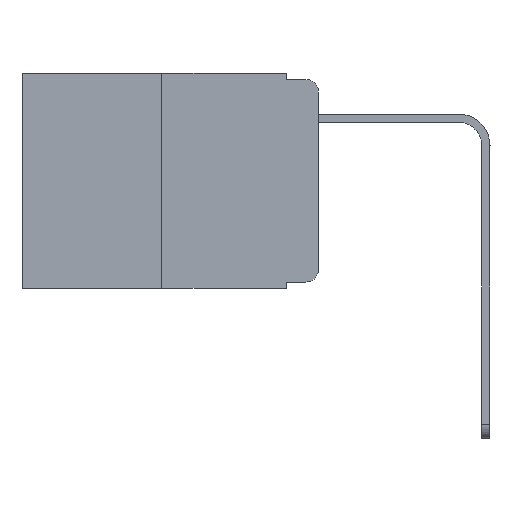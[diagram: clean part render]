
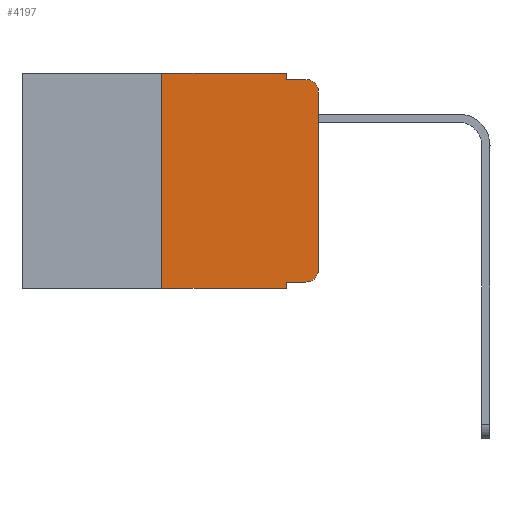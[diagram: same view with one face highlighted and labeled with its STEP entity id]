
A CAD part, left-side view. The second image highlights one B-rep face of the part: STEP entity #4197.
In plain terms, the highlighted planar face has unit normal (-1, 0, 0).
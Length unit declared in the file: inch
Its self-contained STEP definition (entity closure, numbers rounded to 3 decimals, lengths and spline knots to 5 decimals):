
#75 = VERTEX_POINT ( 'NONE', #1834 ) ;
#324 = VERTEX_POINT ( 'NONE', #2211 ) ;
#340 = ORIENTED_EDGE ( 'NONE', *, *, #642, .T. ) ;
#403 = DIRECTION ( 'NONE',  ( -1., 0., 0. ) ) ;
#424 = DIRECTION ( 'NONE',  ( 0., 0., -1. ) ) ;
#642 = EDGE_CURVE ( 'NONE', #324, #2455, #707, .T. ) ;
#693 = CARTESIAN_POINT ( 'NONE',  ( 0., 0.02, -0.01 ) ) ;
#707 = CIRCLE ( 'NONE', #5364, 0.02 ) ;
#715 = DIRECTION ( 'NONE',  ( 0., 0., 1. ) ) ;
#959 = CARTESIAN_POINT ( 'NONE',  ( 0., 0.25, 0. ) ) ;
#1216 = VECTOR ( 'NONE', #8042, 39.37008 ) ;
#1323 = DIRECTION ( 'NONE',  ( 0., -1., 0. ) ) ;
#1361 = CARTESIAN_POINT ( 'NONE',  ( 0., 0.473, -0.343 ) ) ;
#1696 = EDGE_CURVE ( 'NONE', #6298, #324, #5935, .T. ) ;
#1725 = VECTOR ( 'NONE', #3395, 39.37008 ) ;
#1813 = VERTEX_POINT ( 'NONE', #959 ) ;
#1834 = CARTESIAN_POINT ( 'NONE',  ( 0., 0.25, -0.343 ) ) ;
#2011 = CARTESIAN_POINT ( 'NONE',  ( 0., 0.25, 0. ) ) ;
#2147 = VERTEX_POINT ( 'NONE', #693 ) ;
#2211 = CARTESIAN_POINT ( 'NONE',  ( 0., 0.02, -0.333 ) ) ;
#2455 = VERTEX_POINT ( 'NONE', #8117 ) ;
#2466 = EDGE_CURVE ( 'NONE', #11154, #2147, #7695, .T. ) ;
#2518 = VERTEX_POINT ( 'NONE', #2877 ) ;
#2546 = LINE ( 'NONE', #7558, #6874 ) ;
#2628 = LINE ( 'NONE', #1361, #7210 ) ;
#2637 = VECTOR ( 'NONE', #4502, 39.37008 ) ;
#2770 = DIRECTION ( 'NONE',  ( 0., 0., -1. ) ) ;
#2814 = CARTESIAN_POINT ( 'NONE',  ( 0., 0.051, -0.01 ) ) ;
#2847 = EDGE_CURVE ( 'NONE', #2455, #2518, #2546, .T. ) ;
#2877 = CARTESIAN_POINT ( 'NONE',  ( 0., 0., -0.03 ) ) ;
#2889 = ORIENTED_EDGE ( 'NONE', *, *, #3405, .T. ) ;
#2985 = PLANE ( 'NONE',  #8732 ) ;
#3023 = LINE ( 'NONE', #6468, #9498 ) ;
#3395 = DIRECTION ( 'NONE',  ( 0., 0., -1. ) ) ;
#3405 = EDGE_CURVE ( 'NONE', #2518, #2147, #7803, .T. ) ;
#3436 = ORIENTED_EDGE ( 'NONE', *, *, #7038, .F. ) ;
#3482 = LINE ( 'NONE', #8579, #1725 ) ;
#3549 = EDGE_CURVE ( 'NONE', #10260, #11154, #3482, .T. ) ;
#3583 = DIRECTION ( 'NONE',  ( 0., 0., -1. ) ) ;
#3618 = VECTOR ( 'NONE', #6072, 39.37008 ) ;
#3817 = CARTESIAN_POINT ( 'NONE',  ( 0., 0.051, -0.01 ) ) ;
#3830 = CARTESIAN_POINT ( 'NONE',  ( 0., 0.473, 0. ) ) ;
#3977 = CARTESIAN_POINT ( 'NONE',  ( 0., 0.051, -0.343 ) ) ;
#4197 = ADVANCED_FACE ( 'NONE', ( #4848 ), #2985, .F. ) ;
#4306 = CARTESIAN_POINT ( 'NONE',  ( 0., 0.051, -0.333 ) ) ;
#4502 = DIRECTION ( 'NONE',  ( 0., 0., 1. ) ) ;
#4652 = LINE ( 'NONE', #2011, #2637 ) ;
#4848 = FACE_OUTER_BOUND ( 'NONE', #9367, .T. ) ;
#4868 = CARTESIAN_POINT ( 'NONE',  ( 0., 0.051, -0.333 ) ) ;
#4989 = ORIENTED_EDGE ( 'NONE', *, *, #2466, .F. ) ;
#5224 = EDGE_CURVE ( 'NONE', #6298, #9052, #8194, .T. ) ;
#5237 = ORIENTED_EDGE ( 'NONE', *, *, #10431, .F. ) ;
#5251 = DIRECTION ( 'NONE',  ( -1., 0., 0. ) ) ;
#5364 = AXIS2_PLACEMENT_3D ( 'NONE', #9698, #5251, #3583 ) ;
#5935 = LINE ( 'NONE', #4306, #3618 ) ;
#6072 = DIRECTION ( 'NONE',  ( 0., -1., 0. ) ) ;
#6174 = VECTOR ( 'NONE', #2770, 39.37008 ) ;
#6298 = VERTEX_POINT ( 'NONE', #4868 ) ;
#6468 = CARTESIAN_POINT ( 'NONE',  ( 0., 0.473, 0. ) ) ;
#6860 = ORIENTED_EDGE ( 'NONE', *, *, #1696, .T. ) ;
#6874 = VECTOR ( 'NONE', #715, 39.37008 ) ;
#7038 = EDGE_CURVE ( 'NONE', #75, #1813, #4652, .T. ) ;
#7210 = VECTOR ( 'NONE', #9217, 39.37008 ) ;
#7366 = ORIENTED_EDGE ( 'NONE', *, *, #2847, .T. ) ;
#7558 = CARTESIAN_POINT ( 'NONE',  ( 0., 0., 0. ) ) ;
#7695 = LINE ( 'NONE', #2814, #1216 ) ;
#7803 = CIRCLE ( 'NONE', #8286, 0.02 ) ;
#7929 = CARTESIAN_POINT ( 'NONE',  ( 0., 0.051, 0. ) ) ;
#7945 = CARTESIAN_POINT ( 'NONE',  ( 0., 0.051, 0. ) ) ;
#8037 = CARTESIAN_POINT ( 'NONE',  ( 0., 0.02, -0.03 ) ) ;
#8042 = DIRECTION ( 'NONE',  ( 0., -1., 0. ) ) ;
#8117 = CARTESIAN_POINT ( 'NONE',  ( 0., 0., -0.313 ) ) ;
#8194 = LINE ( 'NONE', #7929, #6174 ) ;
#8247 = EDGE_CURVE ( 'NONE', #75, #9052, #2628, .T. ) ;
#8286 = AXIS2_PLACEMENT_3D ( 'NONE', #8037, #403, #9783 ) ;
#8561 = ORIENTED_EDGE ( 'NONE', *, *, #8247, .T. ) ;
#8579 = CARTESIAN_POINT ( 'NONE',  ( 0., 0.051, 0. ) ) ;
#8732 = AXIS2_PLACEMENT_3D ( 'NONE', #3830, #10673, #424 ) ;
#9052 = VERTEX_POINT ( 'NONE', #3977 ) ;
#9217 = DIRECTION ( 'NONE',  ( 0., -1., 0. ) ) ;
#9367 = EDGE_LOOP ( 'NONE', ( #7366, #2889, #4989, #10373, #5237, #3436, #8561, #9496, #6860, #340 ) ) ;
#9496 = ORIENTED_EDGE ( 'NONE', *, *, #5224, .F. ) ;
#9498 = VECTOR ( 'NONE', #1323, 39.37008 ) ;
#9698 = CARTESIAN_POINT ( 'NONE',  ( 0., 0.02, -0.313 ) ) ;
#9783 = DIRECTION ( 'NONE',  ( 0., 0., -1. ) ) ;
#10260 = VERTEX_POINT ( 'NONE', #7945 ) ;
#10373 = ORIENTED_EDGE ( 'NONE', *, *, #3549, .F. ) ;
#10431 = EDGE_CURVE ( 'NONE', #1813, #10260, #3023, .T. ) ;
#10673 = DIRECTION ( 'NONE',  ( 1., 0., 0. ) ) ;
#11154 = VERTEX_POINT ( 'NONE', #3817 ) ;
